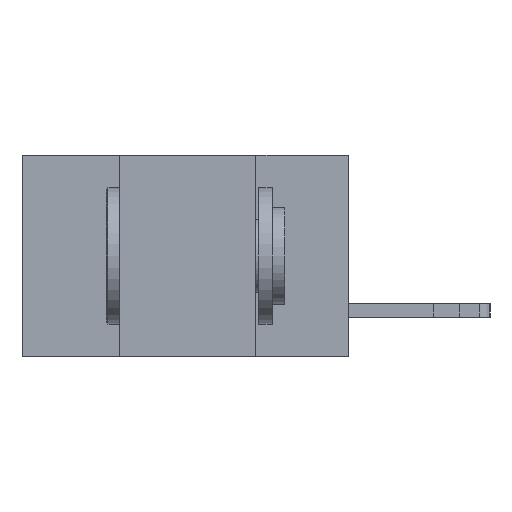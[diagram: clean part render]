
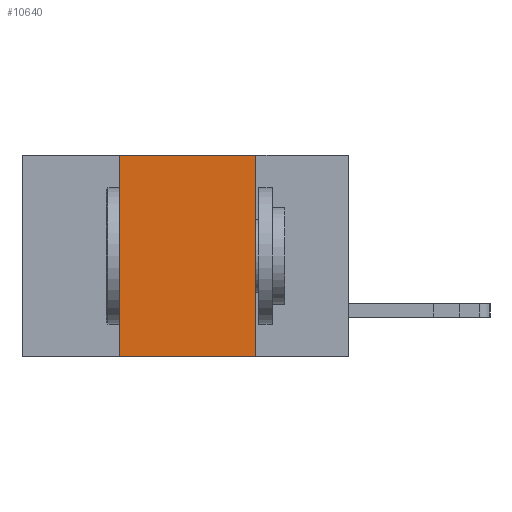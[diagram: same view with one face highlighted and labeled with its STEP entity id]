
A CAD part, left-side view. The second image highlights one B-rep face of the part: STEP entity #10640.
In plain terms, the highlighted planar face has unit normal (-1, 0, 0).
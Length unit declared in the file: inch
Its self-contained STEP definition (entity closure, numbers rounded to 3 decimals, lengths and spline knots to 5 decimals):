
#492 = ORIENTED_EDGE ( 'NONE', *, *, #1758, .T. ) ;
#839 = VECTOR ( 'NONE', #14571, 39.37008 ) ;
#1758 = EDGE_CURVE ( 'NONE', #12876, #22442, #15354, .T. ) ;
#3208 = EDGE_LOOP ( 'NONE', ( #22010, #19928, #3892, #492 ) ) ;
#3519 = LINE ( 'NONE', #12246, #12713 ) ;
#3892 = ORIENTED_EDGE ( 'NONE', *, *, #11892, .F. ) ;
#4209 = EDGE_CURVE ( 'NONE', #5211, #22442, #3519, .T. ) ;
#4749 = VECTOR ( 'NONE', #8527, 39.37008 ) ;
#5113 = EDGE_CURVE ( 'NONE', #12710, #5211, #16331, .T. ) ;
#5211 = VERTEX_POINT ( 'NONE', #6487 ) ;
#5411 = CARTESIAN_POINT ( 'NONE',  ( 0., 0.42, 0. ) ) ;
#5906 = DIRECTION ( 'NONE',  ( 0., -1., 0. ) ) ;
#5982 = CARTESIAN_POINT ( 'NONE',  ( 0., 0.6, 0. ) ) ;
#6487 = CARTESIAN_POINT ( 'NONE',  ( 0., 0.17, 0. ) ) ;
#6768 = PLANE ( 'NONE',  #7479 ) ;
#7479 = AXIS2_PLACEMENT_3D ( 'NONE', #17641, #8580, #21187 ) ;
#8525 = FACE_OUTER_BOUND ( 'NONE', #3208, .T. ) ;
#8527 = DIRECTION ( 'NONE',  ( 0., 0., 1. ) ) ;
#8580 = DIRECTION ( 'NONE',  ( 1., 0., 0. ) ) ;
#9619 = LINE ( 'NONE', #19358, #4749 ) ;
#10486 = DIRECTION ( 'NONE',  ( 0., 0., -1. ) ) ;
#10640 = ADVANCED_FACE ( 'NONE', ( #8525 ), #6768, .F. ) ;
#10688 = CARTESIAN_POINT ( 'NONE',  ( 0., 0.6, -0.37 ) ) ;
#11892 = EDGE_CURVE ( 'NONE', #12876, #12710, #9619, .T. ) ;
#12090 = VECTOR ( 'NONE', #5906, 39.37008 ) ;
#12246 = CARTESIAN_POINT ( 'NONE',  ( 0., 0.17, 0. ) ) ;
#12710 = VERTEX_POINT ( 'NONE', #5411 ) ;
#12713 = VECTOR ( 'NONE', #10486, 39.37008 ) ;
#12876 = VERTEX_POINT ( 'NONE', #16756 ) ;
#14571 = DIRECTION ( 'NONE',  ( 0., -1., 0. ) ) ;
#15354 = LINE ( 'NONE', #10688, #839 ) ;
#16331 = LINE ( 'NONE', #5982, #12090 ) ;
#16756 = CARTESIAN_POINT ( 'NONE',  ( 0., 0.42, -0.37 ) ) ;
#17641 = CARTESIAN_POINT ( 'NONE',  ( 0., 0.6, 0. ) ) ;
#18279 = CARTESIAN_POINT ( 'NONE',  ( 0., 0.17, -0.37 ) ) ;
#19358 = CARTESIAN_POINT ( 'NONE',  ( 0., 0.42, 0. ) ) ;
#19928 = ORIENTED_EDGE ( 'NONE', *, *, #5113, .F. ) ;
#21187 = DIRECTION ( 'NONE',  ( 0., 0., -1. ) ) ;
#22010 = ORIENTED_EDGE ( 'NONE', *, *, #4209, .F. ) ;
#22442 = VERTEX_POINT ( 'NONE', #18279 ) ;
